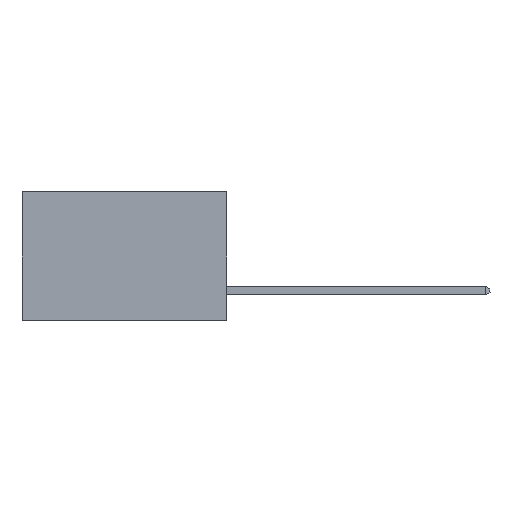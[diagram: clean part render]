
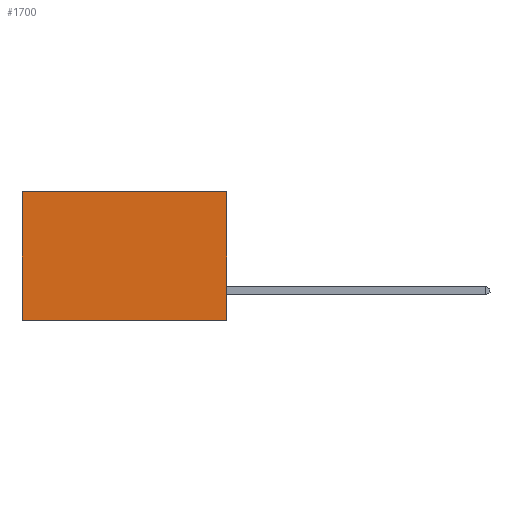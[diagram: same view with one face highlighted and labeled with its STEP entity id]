
A CAD part, left-side view. The second image highlights one B-rep face of the part: STEP entity #1700.
In plain terms, the highlighted planar face has unit normal (-1, 0, 0).
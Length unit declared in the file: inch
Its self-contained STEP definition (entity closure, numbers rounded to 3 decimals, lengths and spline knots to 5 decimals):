
#329 = CARTESIAN_POINT ( 'NONE',  ( 0.277, 0., -0.37 ) ) ;
#408 = DIRECTION ( 'NONE',  ( 0., 1., 0. ) ) ;
#424 = VERTEX_POINT ( 'NONE', #1282 ) ;
#442 = DIRECTION ( 'NONE',  ( 1., 0., 0. ) ) ;
#501 = CARTESIAN_POINT ( 'NONE',  ( 0.277, 0.59, 0. ) ) ;
#508 = LINE ( 'NONE', #1890, #10009 ) ;
#543 = VERTEX_POINT ( 'NONE', #1639 ) ;
#603 = EDGE_LOOP ( 'NONE', ( #2827, #5377, #10160, #5671 ) ) ;
#720 = VECTOR ( 'NONE', #10143, 39.37008 ) ;
#1282 = CARTESIAN_POINT ( 'NONE',  ( 0.277, 0., -0.37 ) ) ;
#1639 = CARTESIAN_POINT ( 'NONE',  ( 0.277, 0.59, -0.37 ) ) ;
#1669 = FACE_OUTER_BOUND ( 'NONE', #603, .T. ) ;
#1700 = ADVANCED_FACE ( 'NONE', ( #1669 ), #6338, .F. ) ;
#1890 = CARTESIAN_POINT ( 'NONE',  ( 0.277, 0.59, -0.37 ) ) ;
#2747 = CARTESIAN_POINT ( 'NONE',  ( 0.277, 0., 0. ) ) ;
#2827 = ORIENTED_EDGE ( 'NONE', *, *, #9135, .T. ) ;
#3568 = VERTEX_POINT ( 'NONE', #501 ) ;
#4096 = AXIS2_PLACEMENT_3D ( 'NONE', #329, #442, #6173 ) ;
#4322 = VECTOR ( 'NONE', #408, 39.37008 ) ;
#4886 = CARTESIAN_POINT ( 'NONE',  ( 0.277, 0., -0.37 ) ) ;
#5377 = ORIENTED_EDGE ( 'NONE', *, *, #10795, .F. ) ;
#5671 = ORIENTED_EDGE ( 'NONE', *, *, #8785, .T. ) ;
#5847 = DIRECTION ( 'NONE',  ( 0., 0., -1. ) ) ;
#6173 = DIRECTION ( 'NONE',  ( 0., 0., -1. ) ) ;
#6338 = PLANE ( 'NONE',  #4096 ) ;
#6723 = DIRECTION ( 'NONE',  ( 0., 0., -1. ) ) ;
#6819 = VERTEX_POINT ( 'NONE', #2747 ) ;
#7481 = CARTESIAN_POINT ( 'NONE',  ( 0.277, 0., -0.37 ) ) ;
#7654 = LINE ( 'NONE', #4886, #12040 ) ;
#8659 = LINE ( 'NONE', #7481, #720 ) ;
#8785 = EDGE_CURVE ( 'NONE', #6819, #3568, #8894, .T. ) ;
#8894 = LINE ( 'NONE', #8989, #4322 ) ;
#8989 = CARTESIAN_POINT ( 'NONE',  ( 0.277, 0., 0. ) ) ;
#9135 = EDGE_CURVE ( 'NONE', #3568, #543, #508, .T. ) ;
#9147 = EDGE_CURVE ( 'NONE', #6819, #424, #7654, .T. ) ;
#10009 = VECTOR ( 'NONE', #6723, 39.37008 ) ;
#10143 = DIRECTION ( 'NONE',  ( 0., 1., 0. ) ) ;
#10160 = ORIENTED_EDGE ( 'NONE', *, *, #9147, .F. ) ;
#10795 = EDGE_CURVE ( 'NONE', #424, #543, #8659, .T. ) ;
#12040 = VECTOR ( 'NONE', #5847, 39.37008 ) ;
